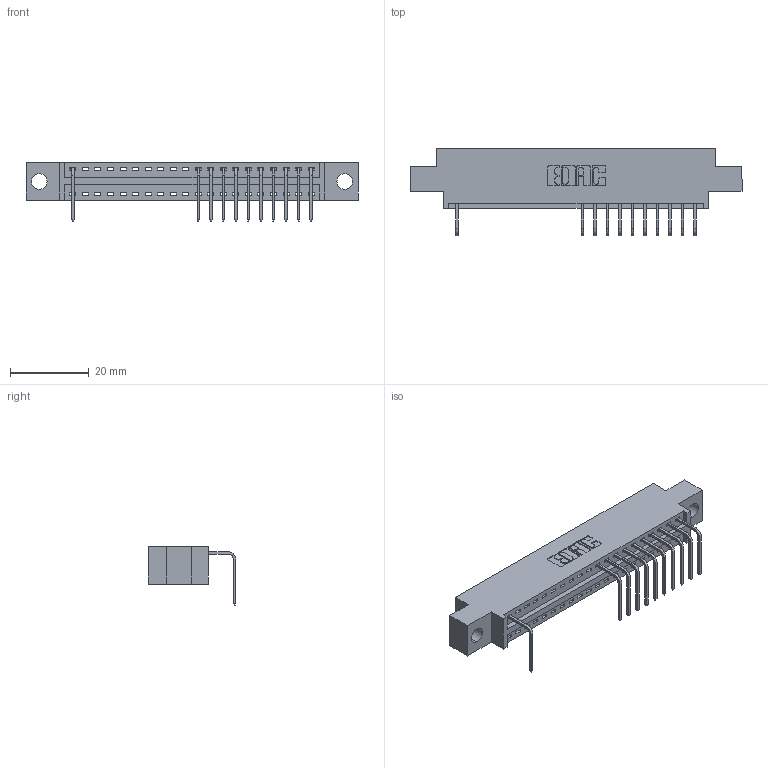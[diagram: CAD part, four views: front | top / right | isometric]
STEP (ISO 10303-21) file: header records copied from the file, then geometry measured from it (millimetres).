
FILE_DESCRIPTION (( 'STEP AP203' ), '1' );
FILE_NAME ('346-020-558-604.STEP', '2018-08-20T22:12:06', ( '' ), ( '' ), 'SwSTEP 2.0', 'SolidWorks 2016', '' );
FILE_SCHEMA (( 'CONFIG_CONTROL_DESIGN' ));
Length unit declared in the file: inch
Products named in the file (3): 346 Part_0.170 Offset - 0.156 Dia-TH; 345-292-001_558 Tail - 2; 346-020-558-604
Assembly tree (12 placements, depth 2):
  346-020-558-604
    346 Part_0.170 Offset - 0.156 Dia-TH
    345-292-001_558 Tail - 2  x11
Bounding box: 84.07 x 22.16 x 14.73 mm (x, y, z)
Volume: 7587.4 mm3; surface area: 8876 mm2
Topology: 12 solids, 12 shells, 894 faces, 2721 edges, 1798 vertices
Faces by surface type: plane 632, cylinder 262
Entity records: 15305 total; most frequent: CARTESIAN_POINT 2679, ORIENTED_EDGE 2642, DIRECTION 2379, EDGE_CURVE 1321, VECTOR 1109, LINE 1109, VERTEX_POINT 878, AXIS2_PLACEMENT_3D 635
